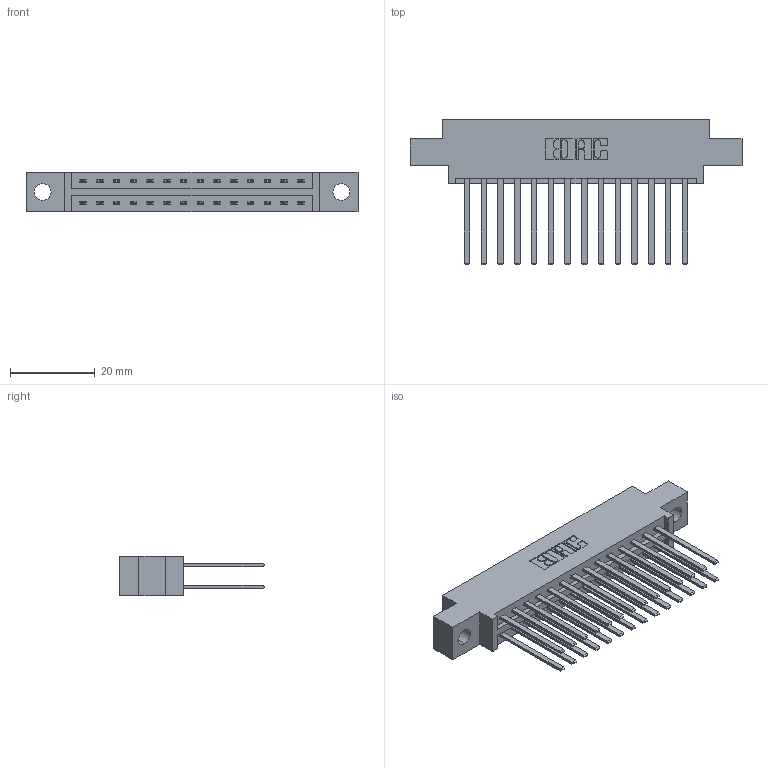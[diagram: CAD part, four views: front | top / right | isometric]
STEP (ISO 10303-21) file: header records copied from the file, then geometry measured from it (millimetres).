
FILE_DESCRIPTION (( 'STEP AP203' ), '1' );
FILE_NAME ('337-028-544-804.STEP', '2018-08-06T11:33:23', ( '' ), ( '' ), 'SwSTEP 2.0', 'SolidWorks 2016', '' );
FILE_SCHEMA (( 'CONFIG_CONTROL_DESIGN' ));
Length unit declared in the file: inch
Products named in the file (3): 345-292-001_345-293-144; 337-028-544-804; 337 Part_0.170 Offset - 0.156 Dia-TH
Assembly tree (29 placements, depth 2):
  337-028-544-804
    337 Part_0.170 Offset - 0.156 Dia-TH
    345-292-001_345-293-144  x28
Bounding box: 78.49 x 34.3 x 9.4 mm (x, y, z)
Volume: 8085.9 mm3; surface area: 10056.6 mm2
Topology: 29 solids, 29 shells, 1462 faces, 4327 edges, 2846 vertices
Faces by surface type: plane 1026, cylinder 436
Entity records: 14427 total; most frequent: CARTESIAN_POINT 2454, ORIENTED_EDGE 2390, DIRECTION 2135, EDGE_CURVE 1195, VECTOR 1071, LINE 1071, VERTEX_POINT 794, AXIS2_PLACEMENT_3D 532
